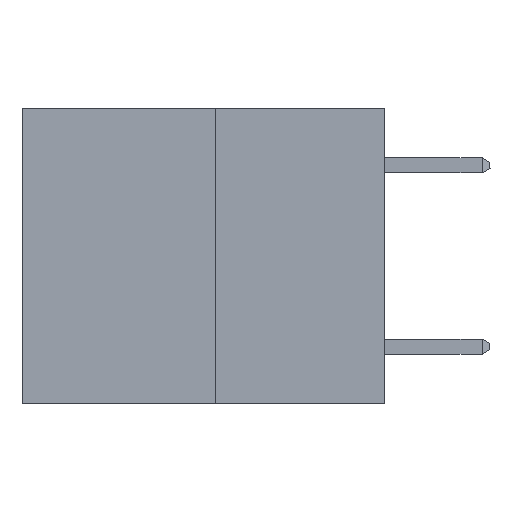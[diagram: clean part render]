
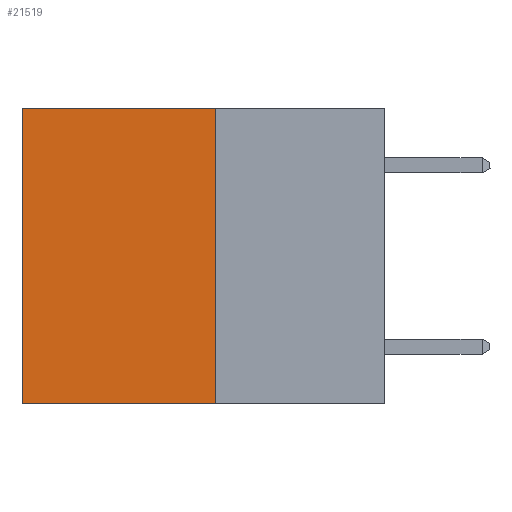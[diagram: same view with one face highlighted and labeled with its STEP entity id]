
A CAD part, left-side view. The second image highlights one B-rep face of the part: STEP entity #21519.
In plain terms, the highlighted planar face has unit normal (-1, 0, 0).
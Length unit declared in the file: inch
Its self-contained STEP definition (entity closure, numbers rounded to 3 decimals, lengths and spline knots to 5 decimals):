
#1218 = VERTEX_POINT ( 'NONE', #13756 ) ;
#1987 = VERTEX_POINT ( 'NONE', #15264 ) ;
#4303 = DIRECTION ( 'NONE',  ( 0., 1., 0. ) ) ;
#4375 = LINE ( 'NONE', #5434, #10799 ) ;
#4999 = VECTOR ( 'NONE', #11169, 39.37008 ) ;
#5361 = VECTOR ( 'NONE', #4303, 39.37008 ) ;
#5434 = CARTESIAN_POINT ( 'NONE',  ( 0.3165, 0.28, -0.49 ) ) ;
#5968 = VERTEX_POINT ( 'NONE', #8968 ) ;
#6177 = EDGE_CURVE ( 'NONE', #11069, #5968, #19605, .T. ) ;
#6833 = ORIENTED_EDGE ( 'NONE', *, *, #7097, .T. ) ;
#6848 = DIRECTION ( 'NONE',  ( 0., 0., -1. ) ) ;
#7097 = EDGE_CURVE ( 'NONE', #1218, #1987, #11394, .T. ) ;
#8968 = CARTESIAN_POINT ( 'NONE',  ( 0.3165, 0.28, -0.49 ) ) ;
#8980 = VECTOR ( 'NONE', #18691, 39.37008 ) ;
#10013 = EDGE_CURVE ( 'NONE', #11069, #1218, #10445, .T. ) ;
#10445 = LINE ( 'NONE', #16302, #5361 ) ;
#10799 = VECTOR ( 'NONE', #20486, 39.37008 ) ;
#11069 = VERTEX_POINT ( 'NONE', #13017 ) ;
#11169 = DIRECTION ( 'NONE',  ( 0., 0., -1. ) ) ;
#11394 = LINE ( 'NONE', #18624, #8980 ) ;
#12767 = ORIENTED_EDGE ( 'NONE', *, *, #6177, .F. ) ;
#13017 = CARTESIAN_POINT ( 'NONE',  ( 0.3165, 0.28, 0. ) ) ;
#13168 = ORIENTED_EDGE ( 'NONE', *, *, #20432, .F. ) ;
#13756 = CARTESIAN_POINT ( 'NONE',  ( 0.3165, 0.6, 0. ) ) ;
#14623 = CARTESIAN_POINT ( 'NONE',  ( 0.3165, 0.28, -0.49 ) ) ;
#15238 = FACE_OUTER_BOUND ( 'NONE', #15595, .T. ) ;
#15264 = CARTESIAN_POINT ( 'NONE',  ( 0.3165, 0.6, -0.49 ) ) ;
#15595 = EDGE_LOOP ( 'NONE', ( #6833, #13168, #12767, #19934 ) ) ;
#16302 = CARTESIAN_POINT ( 'NONE',  ( 0.3165, 0.28, 0. ) ) ;
#17012 = DIRECTION ( 'NONE',  ( 1., 0., 0. ) ) ;
#18624 = CARTESIAN_POINT ( 'NONE',  ( 0.3165, 0.6, -0.49 ) ) ;
#18691 = DIRECTION ( 'NONE',  ( 0., 0., -1. ) ) ;
#18996 = PLANE ( 'NONE',  #19821 ) ;
#19605 = LINE ( 'NONE', #14623, #4999 ) ;
#19821 = AXIS2_PLACEMENT_3D ( 'NONE', #20686, #17012, #6848 ) ;
#19934 = ORIENTED_EDGE ( 'NONE', *, *, #10013, .T. ) ;
#20432 = EDGE_CURVE ( 'NONE', #5968, #1987, #4375, .T. ) ;
#20486 = DIRECTION ( 'NONE',  ( 0., 1., 0. ) ) ;
#20686 = CARTESIAN_POINT ( 'NONE',  ( 0.3165, 0.28, -0.49 ) ) ;
#21519 = ADVANCED_FACE ( 'NONE', ( #15238 ), #18996, .F. ) ;
